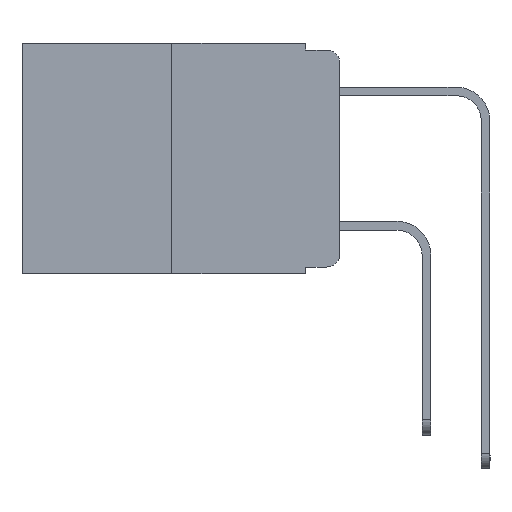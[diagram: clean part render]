
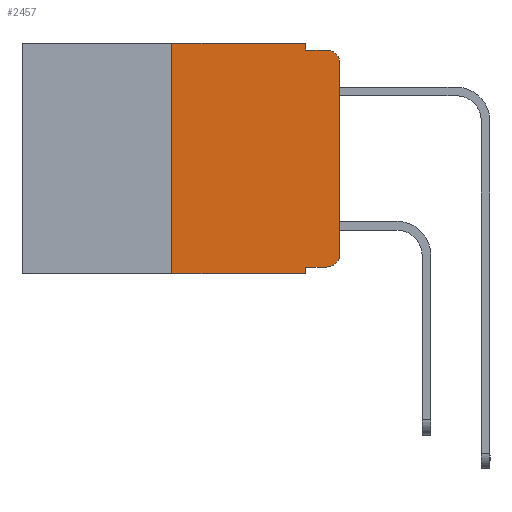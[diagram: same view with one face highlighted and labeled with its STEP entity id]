
A CAD part, left-side view. The second image highlights one B-rep face of the part: STEP entity #2457.
In plain terms, the highlighted planar face has unit normal (-1, 0, 0).
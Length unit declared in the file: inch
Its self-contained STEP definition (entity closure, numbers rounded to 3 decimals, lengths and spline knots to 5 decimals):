
#84 = VECTOR ( 'NONE', #373, 39.37008 ) ;
#113 = LINE ( 'NONE', #6153, #7683 ) ;
#126 = CARTESIAN_POINT ( 'NONE',  ( 0., 0.051, -0.333 ) ) ;
#373 = DIRECTION ( 'NONE',  ( 0., -1., 0. ) ) ;
#389 = DIRECTION ( 'NONE',  ( 1., 0., 0. ) ) ;
#485 = DIRECTION ( 'NONE',  ( 0., 0., -1. ) ) ;
#914 = VERTEX_POINT ( 'NONE', #9036 ) ;
#1197 = DIRECTION ( 'NONE',  ( 0., 0., -1. ) ) ;
#1198 = CARTESIAN_POINT ( 'NONE',  ( 0., 0.473, 0. ) ) ;
#1293 = CARTESIAN_POINT ( 'NONE',  ( 0., 0.051, -0.01 ) ) ;
#1305 = VERTEX_POINT ( 'NONE', #2788 ) ;
#1523 = DIRECTION ( 'NONE',  ( 0., -1., 0. ) ) ;
#1614 = VERTEX_POINT ( 'NONE', #8478 ) ;
#2017 = VECTOR ( 'NONE', #485, 39.37008 ) ;
#2177 = ORIENTED_EDGE ( 'NONE', *, *, #6355, .F. ) ;
#2217 = DIRECTION ( 'NONE',  ( -1., 0., 0. ) ) ;
#2381 = CARTESIAN_POINT ( 'NONE',  ( 0., 0.473, 0. ) ) ;
#2385 = CARTESIAN_POINT ( 'NONE',  ( 0., 0.051, 0. ) ) ;
#2457 = ADVANCED_FACE ( 'NONE', ( #9498 ), #12540, .F. ) ;
#2698 = VECTOR ( 'NONE', #6207, 39.37008 ) ;
#2788 = CARTESIAN_POINT ( 'NONE',  ( 0., 0.051, 0. ) ) ;
#2896 = CARTESIAN_POINT ( 'NONE',  ( 0., 0., -0.03 ) ) ;
#3003 = VERTEX_POINT ( 'NONE', #10751 ) ;
#3371 = CARTESIAN_POINT ( 'NONE',  ( 0., 0.051, -0.343 ) ) ;
#3744 = EDGE_CURVE ( 'NONE', #1614, #914, #13029, .T. ) ;
#3893 = CARTESIAN_POINT ( 'NONE',  ( 0., 0.25, 0. ) ) ;
#4245 = CARTESIAN_POINT ( 'NONE',  ( 0., 0., 0. ) ) ;
#4317 = DIRECTION ( 'NONE',  ( 0., 0., -1. ) ) ;
#5142 = VECTOR ( 'NONE', #10997, 39.37008 ) ;
#5477 = EDGE_CURVE ( 'NONE', #10794, #8847, #9830, .T. ) ;
#5569 = VERTEX_POINT ( 'NONE', #8620 ) ;
#5763 = CARTESIAN_POINT ( 'NONE',  ( 0., 0.051, -0.01 ) ) ;
#5787 = EDGE_LOOP ( 'NONE', ( #6335, #10600, #12623, #7485, #10488, #6083, #10689, #2177, #11103, #11507 ) ) ;
#5926 = DIRECTION ( 'NONE',  ( 0., 0., -1. ) ) ;
#6033 = EDGE_CURVE ( 'NONE', #1614, #9117, #6671, .T. ) ;
#6056 = AXIS2_PLACEMENT_3D ( 'NONE', #7057, #9056, #5926 ) ;
#6083 = ORIENTED_EDGE ( 'NONE', *, *, #3744, .F. ) ;
#6153 = CARTESIAN_POINT ( 'NONE',  ( 0., 0.051, 0. ) ) ;
#6207 = DIRECTION ( 'NONE',  ( 0., -1., 0. ) ) ;
#6335 = ORIENTED_EDGE ( 'NONE', *, *, #7550, .T. ) ;
#6355 = EDGE_CURVE ( 'NONE', #7108, #9117, #9468, .T. ) ;
#6671 = LINE ( 'NONE', #12849, #84 ) ;
#6684 = CARTESIAN_POINT ( 'NONE',  ( 0., 0.051, -0.333 ) ) ;
#7057 = CARTESIAN_POINT ( 'NONE',  ( 0., 0.02, -0.03 ) ) ;
#7108 = VERTEX_POINT ( 'NONE', #126 ) ;
#7345 = CARTESIAN_POINT ( 'NONE',  ( 0., 0.02, -0.01 ) ) ;
#7440 = CARTESIAN_POINT ( 'NONE',  ( 0., 0.02, -0.313 ) ) ;
#7485 = ORIENTED_EDGE ( 'NONE', *, *, #10378, .F. ) ;
#7550 = EDGE_CURVE ( 'NONE', #3003, #9336, #10280, .T. ) ;
#7554 = DIRECTION ( 'NONE',  ( 0., -1., 0. ) ) ;
#7683 = VECTOR ( 'NONE', #4317, 39.37008 ) ;
#7758 = LINE ( 'NONE', #6684, #9329 ) ;
#8478 = CARTESIAN_POINT ( 'NONE',  ( 0., 0.25, -0.343 ) ) ;
#8620 = CARTESIAN_POINT ( 'NONE',  ( 0., 0.02, -0.333 ) ) ;
#8802 = VECTOR ( 'NONE', #9221, 39.37008 ) ;
#8847 = VERTEX_POINT ( 'NONE', #7345 ) ;
#8973 = VECTOR ( 'NONE', #1523, 39.37008 ) ;
#9036 = CARTESIAN_POINT ( 'NONE',  ( 0., 0.25, 0. ) ) ;
#9056 = DIRECTION ( 'NONE',  ( -1., 0., 0. ) ) ;
#9061 = AXIS2_PLACEMENT_3D ( 'NONE', #7440, #2217, #1197 ) ;
#9117 = VERTEX_POINT ( 'NONE', #3371 ) ;
#9221 = DIRECTION ( 'NONE',  ( 0., 0., 1. ) ) ;
#9329 = VECTOR ( 'NONE', #7554, 39.37008 ) ;
#9336 = VERTEX_POINT ( 'NONE', #2896 ) ;
#9378 = DIRECTION ( 'NONE',  ( 0., 0., -1. ) ) ;
#9443 = EDGE_CURVE ( 'NONE', #9336, #8847, #12260, .T. ) ;
#9468 = LINE ( 'NONE', #2385, #2017 ) ;
#9498 = FACE_OUTER_BOUND ( 'NONE', #5787, .T. ) ;
#9697 = CIRCLE ( 'NONE', #9061, 0.02 ) ;
#9811 = AXIS2_PLACEMENT_3D ( 'NONE', #1198, #389, #9378 ) ;
#9830 = LINE ( 'NONE', #5763, #8973 ) ;
#10280 = LINE ( 'NONE', #4245, #8802 ) ;
#10378 = EDGE_CURVE ( 'NONE', #1305, #10794, #113, .T. ) ;
#10488 = ORIENTED_EDGE ( 'NONE', *, *, #10926, .F. ) ;
#10600 = ORIENTED_EDGE ( 'NONE', *, *, #9443, .T. ) ;
#10689 = ORIENTED_EDGE ( 'NONE', *, *, #6033, .T. ) ;
#10751 = CARTESIAN_POINT ( 'NONE',  ( 0., 0., -0.313 ) ) ;
#10794 = VERTEX_POINT ( 'NONE', #1293 ) ;
#10926 = EDGE_CURVE ( 'NONE', #914, #1305, #11282, .T. ) ;
#10997 = DIRECTION ( 'NONE',  ( 0., 0., 1. ) ) ;
#11103 = ORIENTED_EDGE ( 'NONE', *, *, #12948, .T. ) ;
#11282 = LINE ( 'NONE', #2381, #2698 ) ;
#11349 = EDGE_CURVE ( 'NONE', #5569, #3003, #9697, .T. ) ;
#11507 = ORIENTED_EDGE ( 'NONE', *, *, #11349, .T. ) ;
#12260 = CIRCLE ( 'NONE', #6056, 0.02 ) ;
#12540 = PLANE ( 'NONE',  #9811 ) ;
#12623 = ORIENTED_EDGE ( 'NONE', *, *, #5477, .F. ) ;
#12849 = CARTESIAN_POINT ( 'NONE',  ( 0., 0.473, -0.343 ) ) ;
#12948 = EDGE_CURVE ( 'NONE', #7108, #5569, #7758, .T. ) ;
#13029 = LINE ( 'NONE', #3893, #5142 ) ;
